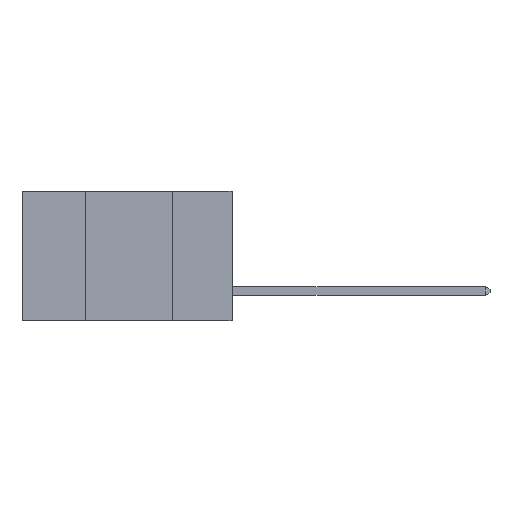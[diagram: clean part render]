
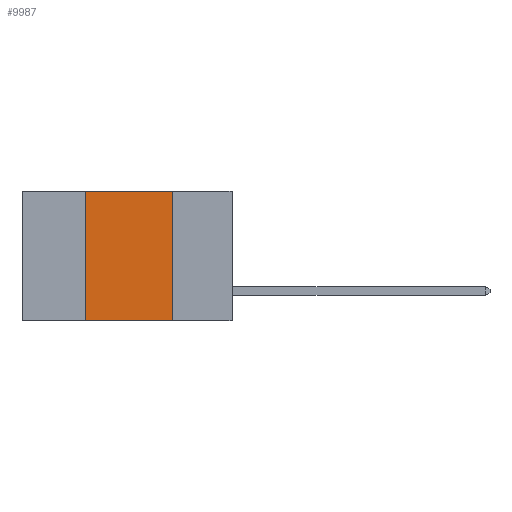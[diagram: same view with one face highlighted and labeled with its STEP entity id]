
A CAD part, left-side view. The second image highlights one B-rep face of the part: STEP entity #9987.
In plain terms, the highlighted planar face has unit normal (-1, 0, 0).
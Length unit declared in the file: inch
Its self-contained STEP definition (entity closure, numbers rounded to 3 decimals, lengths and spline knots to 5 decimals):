
#50 = FACE_OUTER_BOUND ( 'NONE', #6091, .T. ) ;
#292 = VERTEX_POINT ( 'NONE', #6422 ) ;
#494 = VERTEX_POINT ( 'NONE', #754 ) ;
#754 = CARTESIAN_POINT ( 'NONE',  ( 0., 0.42, 0. ) ) ;
#846 = CARTESIAN_POINT ( 'NONE',  ( 0., 0.6, 0. ) ) ;
#1015 = DIRECTION ( 'NONE',  ( 1., 0., 0. ) ) ;
#1351 = VERTEX_POINT ( 'NONE', #8911 ) ;
#1730 = VECTOR ( 'NONE', #10466, 39.37008 ) ;
#1745 = VECTOR ( 'NONE', #2844, 39.37008 ) ;
#2813 = AXIS2_PLACEMENT_3D ( 'NONE', #10596, #1015, #7903 ) ;
#2844 = DIRECTION ( 'NONE',  ( 0., -1., 0. ) ) ;
#2980 = CARTESIAN_POINT ( 'NONE',  ( 0., 0.17, 0. ) ) ;
#3975 = DIRECTION ( 'NONE',  ( 0., 0., 1. ) ) ;
#4384 = ORIENTED_EDGE ( 'NONE', *, *, #7018, .F. ) ;
#5066 = PLANE ( 'NONE',  #2813 ) ;
#5149 = ORIENTED_EDGE ( 'NONE', *, *, #9661, .T. ) ;
#5264 = EDGE_CURVE ( 'NONE', #494, #7570, #9443, .T. ) ;
#5339 = ORIENTED_EDGE ( 'NONE', *, *, #12010, .F. ) ;
#5508 = CARTESIAN_POINT ( 'NONE',  ( 0., 0.6, -0.37 ) ) ;
#6091 = EDGE_LOOP ( 'NONE', ( #5339, #9690, #4384, #5149 ) ) ;
#6422 = CARTESIAN_POINT ( 'NONE',  ( 0., 0.42, -0.37 ) ) ;
#6489 = VECTOR ( 'NONE', #8287, 39.37008 ) ;
#6558 = VECTOR ( 'NONE', #3975, 39.37008 ) ;
#7018 = EDGE_CURVE ( 'NONE', #292, #494, #11121, .T. ) ;
#7570 = VERTEX_POINT ( 'NONE', #2980 ) ;
#7903 = DIRECTION ( 'NONE',  ( 0., 0., -1. ) ) ;
#8287 = DIRECTION ( 'NONE',  ( 0., -1., 0. ) ) ;
#8911 = CARTESIAN_POINT ( 'NONE',  ( 0., 0.17, -0.37 ) ) ;
#8914 = LINE ( 'NONE', #5508, #6489 ) ;
#9443 = LINE ( 'NONE', #846, #1745 ) ;
#9590 = CARTESIAN_POINT ( 'NONE',  ( 0., 0.17, 0. ) ) ;
#9661 = EDGE_CURVE ( 'NONE', #292, #1351, #8914, .T. ) ;
#9690 = ORIENTED_EDGE ( 'NONE', *, *, #5264, .F. ) ;
#9987 = ADVANCED_FACE ( 'NONE', ( #50 ), #5066, .F. ) ;
#10466 = DIRECTION ( 'NONE',  ( 0., 0., -1. ) ) ;
#10596 = CARTESIAN_POINT ( 'NONE',  ( 0., 0.6, 0. ) ) ;
#11121 = LINE ( 'NONE', #12049, #6558 ) ;
#11561 = LINE ( 'NONE', #9590, #1730 ) ;
#12010 = EDGE_CURVE ( 'NONE', #7570, #1351, #11561, .T. ) ;
#12049 = CARTESIAN_POINT ( 'NONE',  ( 0., 0.42, 0. ) ) ;
